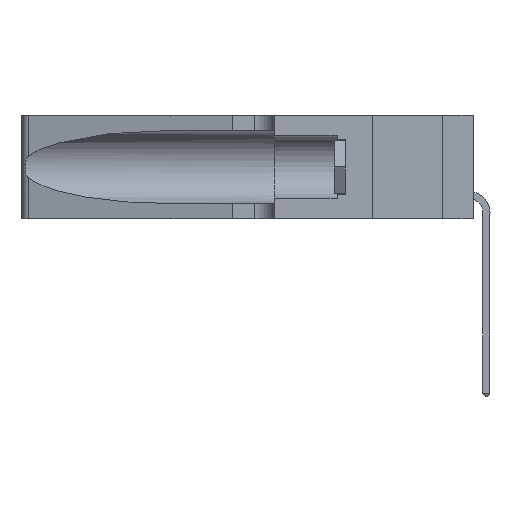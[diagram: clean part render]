
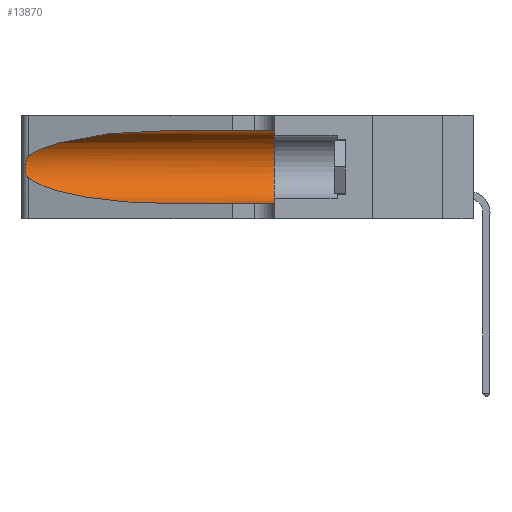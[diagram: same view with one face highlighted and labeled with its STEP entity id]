
A CAD part, left-side view. The second image highlights one B-rep face of the part: STEP entity #13870.
In plain terms, the highlighted cylindrical face has radius 3.308 mm (diameter 6.617 mm), a partial arc.
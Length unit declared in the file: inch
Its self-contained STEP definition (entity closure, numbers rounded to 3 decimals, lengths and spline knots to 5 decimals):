
#343 = EDGE_CURVE ( 'NONE', #13877, #14491, #20629, .T. ) ;
#406 = CARTESIAN_POINT ( 'NONE',  ( 0.25555, 1.22993, 0.14849 ) ) ;
#1689 = ORIENTED_EDGE ( 'NONE', *, *, #17501, .T. ) ;
#3024 = CARTESIAN_POINT ( 'NONE',  ( 0.2373, 1.15595, 0.28018 ) ) ;
#3195 = CARTESIAN_POINT ( 'NONE',  ( 0.25487, 1.22718, 0.22369 ) ) ;
#3633 = CYLINDRICAL_SURFACE ( 'NONE', #5470, 0.13025 ) ;
#4248 = VERTEX_POINT ( 'NONE', #31409 ) ;
#4411 = CARTESIAN_POINT ( 'NONE',  ( 0.1305, 0.35, 0.05475 ) ) ;
#5217 = CARTESIAN_POINT ( 'NONE',  ( 0.26018, 1.23835, 0.19895 ) ) ;
#5321 = CARTESIAN_POINT ( 'NONE',  ( 0.25789, 1.23486, 0.15765 ) ) ;
#5470 = AXIS2_PLACEMENT_3D ( 'NONE', #13360, #13683, #23358 ) ;
#5698 = ORIENTED_EDGE ( 'NONE', *, *, #343, .T. ) ;
#5786 = VECTOR ( 'NONE', #26575, 39.37008 ) ;
#5999 = AXIS2_PLACEMENT_3D ( 'NONE', #25564, #13673, #11008 ) ;
#6545 = VERTEX_POINT ( 'NONE', #6776 ) ;
#6776 = CARTESIAN_POINT ( 'NONE',  ( 0.1305, 0.35, 0.31525 ) ) ;
#7313 = VECTOR ( 'NONE', #27452, 39.37008 ) ;
#8105 = CARTESIAN_POINT ( 'NONE',  ( 0.25487, 1.22718, 0.14631 ) ) ;
#8156 = CARTESIAN_POINT ( 'NONE',  ( 0.1305, 0.72297, 0.31525 ) ) ;
#8356 = CARTESIAN_POINT ( 'NONE',  ( 0.25487, 1.22718, 0.14631 ) ) ;
#8372 = CARTESIAN_POINT ( 'NONE',  ( 0.25487, 1.22718, 0.22369 ) ) ;
#9898 =( BOUNDED_CURVE ( )  B_SPLINE_CURVE ( 3, ( #8156, #12935, #3024, #22476 ),
 .UNSPECIFIED., .F., .F. ) 
 B_SPLINE_CURVE_WITH_KNOTS ( ( 4, 4 ),
 ( 1.5708, 2.84003 ),
 .UNSPECIFIED. ) 
 CURVE ( )  GEOMETRIC_REPRESENTATION_ITEM ( )  RATIONAL_B_SPLINE_CURVE ( ( 1., 0.87, 0.87, 1. ) ) 
 REPRESENTATION_ITEM ( '' )  );
#10336 = CARTESIAN_POINT ( 'NONE',  ( 0.18966, 0.96281, 0.05475 ) ) ;
#10350 = CARTESIAN_POINT ( 'NONE',  ( 0.25555, 1.22994, 0.2215 ) ) ;
#10458 = CARTESIAN_POINT ( 'NONE',  ( 0.1305, 1.61858, 0.31525 ) ) ;
#11008 = DIRECTION ( 'NONE',  ( 0., 0., 1. ) ) ;
#12935 = CARTESIAN_POINT ( 'NONE',  ( 0.18966, 0.96281, 0.31525 ) ) ;
#13020 = LINE ( 'NONE', #21782, #5786 ) ;
#13360 = CARTESIAN_POINT ( 'NONE',  ( 0.1305, 1.61858, 0.185 ) ) ;
#13673 = DIRECTION ( 'NONE',  ( 0., 1., 0. ) ) ;
#13683 = DIRECTION ( 'NONE',  ( 0., -1., 0. ) ) ;
#13870 = ADVANCED_FACE ( 'NONE', ( #16205 ), #3633, .F. ) ;
#13877 = VERTEX_POINT ( 'NONE', #8372 ) ;
#13962 = CARTESIAN_POINT ( 'NONE',  ( 0.1305, 0.72297, 0.31525 ) ) ;
#14491 = VERTEX_POINT ( 'NONE', #8356 ) ;
#14551 = LINE ( 'NONE', #10458, #7313 ) ;
#15308 = CARTESIAN_POINT ( 'NONE',  ( 0.2373, 1.15595, 0.08982 ) ) ;
#15631 = EDGE_CURVE ( 'NONE', #23880, #6545, #14551, .T. ) ;
#15932 =( BOUNDED_CURVE ( )  B_SPLINE_CURVE ( 3, ( #27220, #15308, #10336, #29758 ),
 .UNSPECIFIED., .F., .F. ) 
 B_SPLINE_CURVE_WITH_KNOTS ( ( 4, 4 ),
 ( 3.44316, 4.71239 ),
 .UNSPECIFIED. ) 
 CURVE ( )  GEOMETRIC_REPRESENTATION_ITEM ( )  RATIONAL_B_SPLINE_CURVE ( ( 1., 0.87, 0.87, 1. ) ) 
 REPRESENTATION_ITEM ( '' )  );
#15956 = ORIENTED_EDGE ( 'NONE', *, *, #16854, .T. ) ;
#16205 = FACE_OUTER_BOUND ( 'NONE', #23345, .T. ) ;
#16854 = EDGE_CURVE ( 'NONE', #14491, #4248, #15932, .T. ) ;
#17432 = CARTESIAN_POINT ( 'NONE',  ( 0.25854, 1.2359, 0.20912 ) ) ;
#17501 = EDGE_CURVE ( 'NONE', #4248, #23894, #13020, .T. ) ;
#17644 = CARTESIAN_POINT ( 'NONE',  ( 0.26017, 1.23833, 0.17102 ) ) ;
#19767 = EDGE_CURVE ( 'NONE', #6545, #23894, #28127, .T. ) ;
#19903 = CARTESIAN_POINT ( 'NONE',  ( 0.25639, 1.23184, 0.21858 ) ) ;
#20007 = CARTESIAN_POINT ( 'NONE',  ( 0.25787, 1.23484, 0.2124 ) ) ;
#20222 = CARTESIAN_POINT ( 'NONE',  ( 0.25639, 1.23186, 0.15144 ) ) ;
#20629 = B_SPLINE_CURVE_WITH_KNOTS ( 'NONE', 3,
 ( #3195, #10350, #19903, #20007, #17432, #5217, #24996, #22650, #17644, #27446, #5321, #20222, #406, #8105 ),
 .UNSPECIFIED., .F., .F.,
 ( 4, 2, 2, 2, 2, 2, 4 ),
 ( 0., 0.00027, 0.00053, 0.00107, 0.0016, 0.00187, 0.00214 ),
 .UNSPECIFIED. ) ;
#20669 = ORIENTED_EDGE ( 'NONE', *, *, #19767, .F. ) ;
#21782 = CARTESIAN_POINT ( 'NONE',  ( 0.1305, 1.61858, 0.05475 ) ) ;
#22476 = CARTESIAN_POINT ( 'NONE',  ( 0.25487, 1.22718, 0.22369 ) ) ;
#22650 = CARTESIAN_POINT ( 'NONE',  ( 0.26075, 1.23896, 0.178 ) ) ;
#23345 = EDGE_LOOP ( 'NONE', ( #27526, #5698, #15956, #1689, #20669, #30693 ) ) ;
#23358 = DIRECTION ( 'NONE',  ( 0., 0., -1. ) ) ;
#23880 = VERTEX_POINT ( 'NONE', #13962 ) ;
#23894 = VERTEX_POINT ( 'NONE', #4411 ) ;
#24996 = CARTESIAN_POINT ( 'NONE',  ( 0.26075, 1.23896, 0.19203 ) ) ;
#25564 = CARTESIAN_POINT ( 'NONE',  ( 0.1305, 0.35, 0.185 ) ) ;
#26575 = DIRECTION ( 'NONE',  ( 0., -1., 0. ) ) ;
#27220 = CARTESIAN_POINT ( 'NONE',  ( 0.25487, 1.22718, 0.14631 ) ) ;
#27446 = CARTESIAN_POINT ( 'NONE',  ( 0.25856, 1.23593, 0.16098 ) ) ;
#27452 = DIRECTION ( 'NONE',  ( 0., -1., 0. ) ) ;
#27526 = ORIENTED_EDGE ( 'NONE', *, *, #27982, .T. ) ;
#27982 = EDGE_CURVE ( 'NONE', #23880, #13877, #9898, .T. ) ;
#28127 = CIRCLE ( 'NONE', #5999, 0.13025 ) ;
#29758 = CARTESIAN_POINT ( 'NONE',  ( 0.1305, 0.72297, 0.05475 ) ) ;
#30693 = ORIENTED_EDGE ( 'NONE', *, *, #15631, .F. ) ;
#31409 = CARTESIAN_POINT ( 'NONE',  ( 0.1305, 0.72297, 0.05475 ) ) ;
